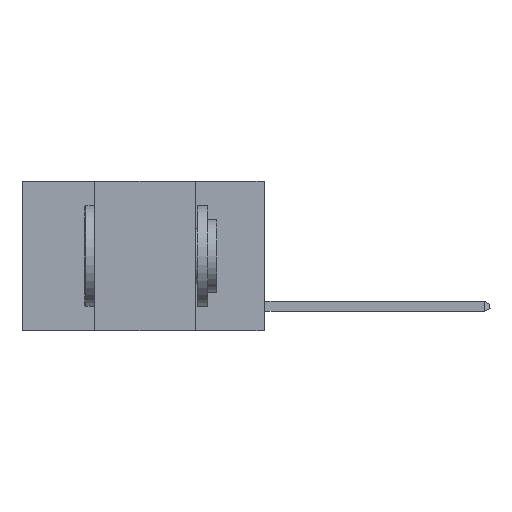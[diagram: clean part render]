
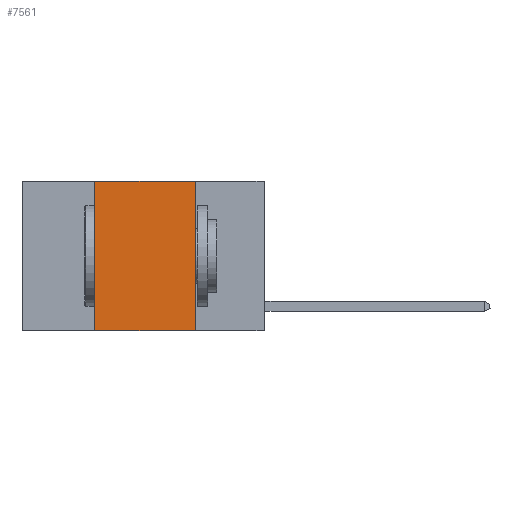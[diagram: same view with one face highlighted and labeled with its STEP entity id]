
A CAD part, left-side view. The second image highlights one B-rep face of the part: STEP entity #7561.
In plain terms, the highlighted planar face has unit normal (-1, 0, 0).
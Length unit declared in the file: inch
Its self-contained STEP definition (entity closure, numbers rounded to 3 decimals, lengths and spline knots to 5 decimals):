
#611 = DIRECTION ( 'NONE',  ( 1., 0., 0. ) ) ;
#629 = CARTESIAN_POINT ( 'NONE',  ( 0., 0.42, 0. ) ) ;
#831 = LINE ( 'NONE', #13019, #8897 ) ;
#1073 = DIRECTION ( 'NONE',  ( 0., -1., 0. ) ) ;
#1886 = VECTOR ( 'NONE', #9852, 39.37008 ) ;
#2276 = ORIENTED_EDGE ( 'NONE', *, *, #9796, .T. ) ;
#2425 = CARTESIAN_POINT ( 'NONE',  ( 0., 0.17, 0. ) ) ;
#2592 = CARTESIAN_POINT ( 'NONE',  ( 0., 0.42, -0.37 ) ) ;
#2772 = VERTEX_POINT ( 'NONE', #7784 ) ;
#2952 = LINE ( 'NONE', #629, #7900 ) ;
#3116 = PLANE ( 'NONE',  #9350 ) ;
#4518 = DIRECTION ( 'NONE',  ( 0., 0., 1. ) ) ;
#5443 = EDGE_CURVE ( 'NONE', #10776, #12222, #2952, .T. ) ;
#7035 = EDGE_CURVE ( 'NONE', #10675, #2772, #12358, .T. ) ;
#7246 = CARTESIAN_POINT ( 'NONE',  ( 0., 0.6, 0. ) ) ;
#7561 = ADVANCED_FACE ( 'NONE', ( #16702 ), #3116, .F. ) ;
#7784 = CARTESIAN_POINT ( 'NONE',  ( 0., 0.17, -0.37 ) ) ;
#7900 = VECTOR ( 'NONE', #4518, 39.37008 ) ;
#7909 = CARTESIAN_POINT ( 'NONE',  ( 0., 0.42, 0. ) ) ;
#7974 = EDGE_LOOP ( 'NONE', ( #12568, #16585, #10067, #2276 ) ) ;
#8845 = LINE ( 'NONE', #16910, #15621 ) ;
#8897 = VECTOR ( 'NONE', #14221, 39.37008 ) ;
#9350 = AXIS2_PLACEMENT_3D ( 'NONE', #7246, #611, #9772 ) ;
#9772 = DIRECTION ( 'NONE',  ( 0., 0., -1. ) ) ;
#9796 = EDGE_CURVE ( 'NONE', #10776, #2772, #831, .T. ) ;
#9852 = DIRECTION ( 'NONE',  ( 0., 0., -1. ) ) ;
#9937 = CARTESIAN_POINT ( 'NONE',  ( 0., 0.17, 0. ) ) ;
#10067 = ORIENTED_EDGE ( 'NONE', *, *, #5443, .F. ) ;
#10675 = VERTEX_POINT ( 'NONE', #2425 ) ;
#10776 = VERTEX_POINT ( 'NONE', #2592 ) ;
#11257 = EDGE_CURVE ( 'NONE', #12222, #10675, #8845, .T. ) ;
#12222 = VERTEX_POINT ( 'NONE', #7909 ) ;
#12358 = LINE ( 'NONE', #9937, #1886 ) ;
#12568 = ORIENTED_EDGE ( 'NONE', *, *, #7035, .F. ) ;
#13019 = CARTESIAN_POINT ( 'NONE',  ( 0., 0.6, -0.37 ) ) ;
#14221 = DIRECTION ( 'NONE',  ( 0., -1., 0. ) ) ;
#15621 = VECTOR ( 'NONE', #1073, 39.37008 ) ;
#16585 = ORIENTED_EDGE ( 'NONE', *, *, #11257, .F. ) ;
#16702 = FACE_OUTER_BOUND ( 'NONE', #7974, .T. ) ;
#16910 = CARTESIAN_POINT ( 'NONE',  ( 0., 0.6, 0. ) ) ;
